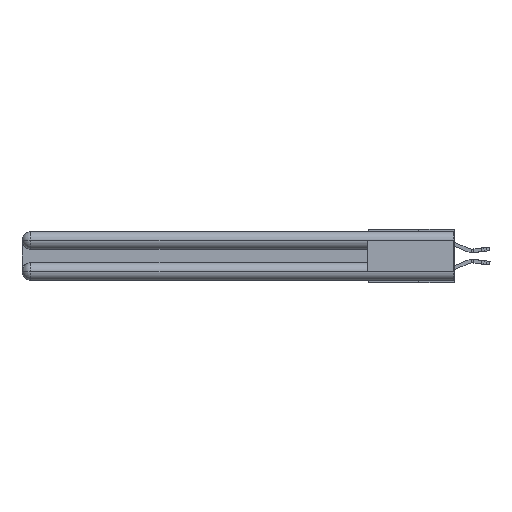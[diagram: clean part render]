
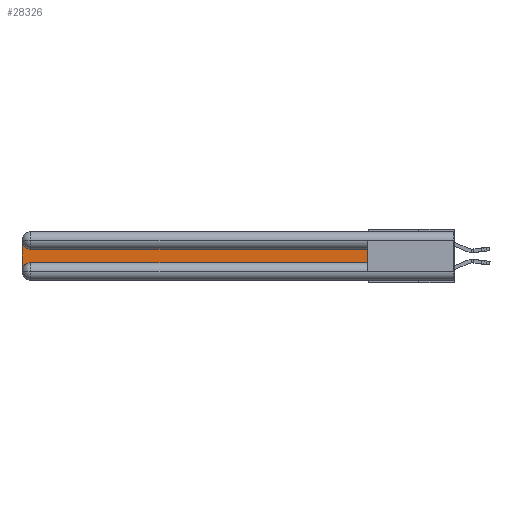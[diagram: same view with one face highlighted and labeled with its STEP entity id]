
A CAD part, left-side view. The second image highlights one B-rep face of the part: STEP entity #28326.
In plain terms, the highlighted planar face has unit normal (-1, 0, 0).
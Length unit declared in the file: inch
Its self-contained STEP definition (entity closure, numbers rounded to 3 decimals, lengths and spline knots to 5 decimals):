
#312 = ORIENTED_EDGE ( 'NONE', *, *, #21449, .T. ) ;
#2958 = DIRECTION ( 'NONE',  ( 0., 0., -1. ) ) ;
#2995 = DIRECTION ( 'NONE',  ( 0., 0., 1. ) ) ;
#3243 = DIRECTION ( 'NONE',  ( 0., -1., 0. ) ) ;
#3875 = ORIENTED_EDGE ( 'NONE', *, *, #20986, .T. ) ;
#4841 = VECTOR ( 'NONE', #2995, 39.37008 ) ;
#5718 = ORIENTED_EDGE ( 'NONE', *, *, #28514, .T. ) ;
#6020 = CARTESIAN_POINT ( 'NONE',  ( 0.075, 3., -0.1225 ) ) ;
#6039 = DIRECTION ( 'NONE',  ( 0., 0., -1. ) ) ;
#8119 = CARTESIAN_POINT ( 'NONE',  ( 0.075, 2.94, -0.0625 ) ) ;
#8511 = EDGE_CURVE ( 'NONE', #11745, #23344, #30962, .T. ) ;
#8548 = EDGE_CURVE ( 'NONE', #31556, #29680, #13870, .T. ) ;
#8596 = CARTESIAN_POINT ( 'NONE',  ( 0.075, 2.94, -0.2775 ) ) ;
#8831 = DIRECTION ( 'NONE',  ( 1., 0., 0. ) ) ;
#9748 = DIRECTION ( 'NONE',  ( 0., 1., 0. ) ) ;
#10787 = DIRECTION ( 'NONE',  ( 0., 0., -1. ) ) ;
#11199 = ORIENTED_EDGE ( 'NONE', *, *, #8511, .T. ) ;
#11396 = CARTESIAN_POINT ( 'NONE',  ( 0.075, 0.6, -0.2175 ) ) ;
#11745 = VERTEX_POINT ( 'NONE', #20570 ) ;
#13043 = VERTEX_POINT ( 'NONE', #27368 ) ;
#13049 = VECTOR ( 'NONE', #2958, 39.37008 ) ;
#13805 = VERTEX_POINT ( 'NONE', #33378 ) ;
#13870 = CIRCLE ( 'NONE', #30563, 0.06 ) ;
#13920 = CARTESIAN_POINT ( 'NONE',  ( 0.075, 3., -0.2175 ) ) ;
#14297 = EDGE_LOOP ( 'NONE', ( #5718, #11199, #17710, #18081, #3875, #312 ) ) ;
#15894 = LINE ( 'NONE', #23649, #16348 ) ;
#16348 = VECTOR ( 'NONE', #9748, 39.37008 ) ;
#16498 = DIRECTION ( 'NONE',  ( 1., 0., 0. ) ) ;
#17386 = LINE ( 'NONE', #13920, #13049 ) ;
#17710 = ORIENTED_EDGE ( 'NONE', *, *, #32080, .T. ) ;
#18081 = ORIENTED_EDGE ( 'NONE', *, *, #8548, .T. ) ;
#19647 = LINE ( 'NONE', #33625, #4841 ) ;
#19804 = DIRECTION ( 'NONE',  ( 1., 0., 0. ) ) ;
#20152 = PLANE ( 'NONE',  #28697 ) ;
#20570 = CARTESIAN_POINT ( 'NONE',  ( 0.075, 2.94, -0.1225 ) ) ;
#20986 = EDGE_CURVE ( 'NONE', #29680, #13805, #24456, .T. ) ;
#21169 = AXIS2_PLACEMENT_3D ( 'NONE', #8119, #16498, #10787 ) ;
#21449 = EDGE_CURVE ( 'NONE', #13805, #13043, #19647, .T. ) ;
#23344 = VERTEX_POINT ( 'NONE', #32828 ) ;
#23649 = CARTESIAN_POINT ( 'NONE',  ( 0.075, 0.6, -0.1225 ) ) ;
#24456 = LINE ( 'NONE', #11396, #25335 ) ;
#25335 = VECTOR ( 'NONE', #3243, 39.37008 ) ;
#27367 = CARTESIAN_POINT ( 'NONE',  ( 0.075, 2.94, -0.2175 ) ) ;
#27368 = CARTESIAN_POINT ( 'NONE',  ( 0.075, 0.6, -0.1225 ) ) ;
#28326 = ADVANCED_FACE ( 'NONE', ( #33448 ), #20152, .F. ) ;
#28488 = DIRECTION ( 'NONE',  ( 0., 0., -1. ) ) ;
#28514 = EDGE_CURVE ( 'NONE', #13043, #11745, #15894, .T. ) ;
#28697 = AXIS2_PLACEMENT_3D ( 'NONE', #6020, #8831, #28488 ) ;
#29680 = VERTEX_POINT ( 'NONE', #27367 ) ;
#30563 = AXIS2_PLACEMENT_3D ( 'NONE', #8596, #19804, #6039 ) ;
#30962 = CIRCLE ( 'NONE', #21169, 0.06 ) ;
#31556 = VERTEX_POINT ( 'NONE', #34849 ) ;
#32080 = EDGE_CURVE ( 'NONE', #23344, #31556, #17386, .T. ) ;
#32828 = CARTESIAN_POINT ( 'NONE',  ( 0.075, 3., -0.0625 ) ) ;
#33378 = CARTESIAN_POINT ( 'NONE',  ( 0.075, 0.6, -0.2175 ) ) ;
#33448 = FACE_OUTER_BOUND ( 'NONE', #14297, .T. ) ;
#33625 = CARTESIAN_POINT ( 'NONE',  ( 0.075, 0.6, -0.2175 ) ) ;
#34849 = CARTESIAN_POINT ( 'NONE',  ( 0.075, 3., -0.2775 ) ) ;
